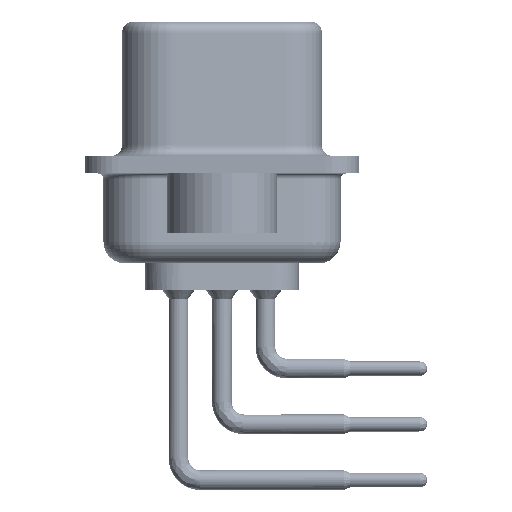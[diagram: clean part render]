
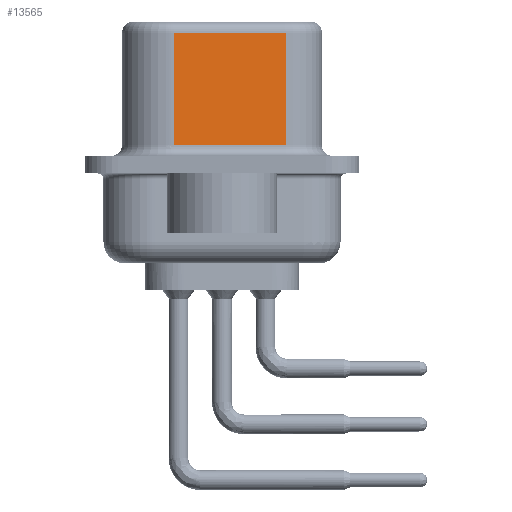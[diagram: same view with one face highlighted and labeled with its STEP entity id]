
A CAD part, left-side view. The second image highlights one B-rep face of the part: STEP entity #13565.
In plain terms, the highlighted planar face has unit normal (-0.985, -0.174, 0).
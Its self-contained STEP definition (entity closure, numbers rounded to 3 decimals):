
#159 = DIRECTION ( 'NONE',  ( 0., 0., -1. ) ) ;
#437 = CARTESIAN_POINT ( 'NONE',  ( 4.58, -2.897, 0.9 ) ) ;
#1012 = DIRECTION ( 'NONE',  ( -0.174, 0.985, 0. ) ) ;
#3206 = CARTESIAN_POINT ( 'NONE',  ( 3.68, 2.203, 6.52 ) ) ;
#3670 = LINE ( 'NONE', #29262, #26637 ) ;
#4237 = EDGE_CURVE ( 'NONE', #21598, #29579, #3670, .T. ) ;
#10632 = DIRECTION ( 'NONE',  ( 0., 0., -1. ) ) ;
#10958 = CARTESIAN_POINT ( 'NONE',  ( 3.68, 2.203, 0.9 ) ) ;
#12790 = ORIENTED_EDGE ( 'NONE', *, *, #4237, .T. ) ;
#13123 = VECTOR ( 'NONE', #31615, 1000. ) ;
#13302 = CARTESIAN_POINT ( 'NONE',  ( 4.58, -2.897, 0.9 ) ) ;
#13474 = PLANE ( 'NONE',  #15237 ) ;
#13565 = ADVANCED_FACE ( 'NONE', ( #16830 ), #13474, .F. ) ;
#14105 = LINE ( 'NONE', #437, #13123 ) ;
#14376 = VECTOR ( 'NONE', #159, 1000. ) ;
#14656 = EDGE_CURVE ( 'NONE', #29579, #26545, #22679, .T. ) ;
#15237 = AXIS2_PLACEMENT_3D ( 'NONE', #38397, #19760, #1012 ) ;
#16830 = FACE_OUTER_BOUND ( 'NONE', #33663, .T. ) ;
#18316 = EDGE_CURVE ( 'NONE', #26545, #23606, #14105, .T. ) ;
#18352 = EDGE_CURVE ( 'NONE', #21598, #23606, #37002, .T. ) ;
#19760 = DIRECTION ( 'NONE',  ( 0.985, 0.174, 0. ) ) ;
#20115 = ORIENTED_EDGE ( 'NONE', *, *, #14656, .T. ) ;
#21598 = VERTEX_POINT ( 'NONE', #35559 ) ;
#22233 = CARTESIAN_POINT ( 'NONE',  ( 3.68, 2.203, 6.02 ) ) ;
#22679 = LINE ( 'NONE', #3206, #14376 ) ;
#23606 = VERTEX_POINT ( 'NONE', #13302 ) ;
#26545 = VERTEX_POINT ( 'NONE', #10958 ) ;
#26637 = VECTOR ( 'NONE', #29408, 1000. ) ;
#28753 = VECTOR ( 'NONE', #10632, 1000. ) ;
#29262 = CARTESIAN_POINT ( 'NONE',  ( 4.58, -2.897, 6.02 ) ) ;
#29408 = DIRECTION ( 'NONE',  ( -0.174, 0.985, 0. ) ) ;
#29579 = VERTEX_POINT ( 'NONE', #22233 ) ;
#31615 = DIRECTION ( 'NONE',  ( 0.174, -0.985, 0. ) ) ;
#32442 = CARTESIAN_POINT ( 'NONE',  ( 4.58, -2.897, 6.52 ) ) ;
#32952 = ORIENTED_EDGE ( 'NONE', *, *, #18316, .T. ) ;
#33663 = EDGE_LOOP ( 'NONE', ( #35076, #12790, #20115, #32952 ) ) ;
#35076 = ORIENTED_EDGE ( 'NONE', *, *, #18352, .F. ) ;
#35559 = CARTESIAN_POINT ( 'NONE',  ( 4.58, -2.897, 6.02 ) ) ;
#37002 = LINE ( 'NONE', #32442, #28753 ) ;
#38397 = CARTESIAN_POINT ( 'NONE',  ( 4.58, -2.897, 6.52 ) ) ;
